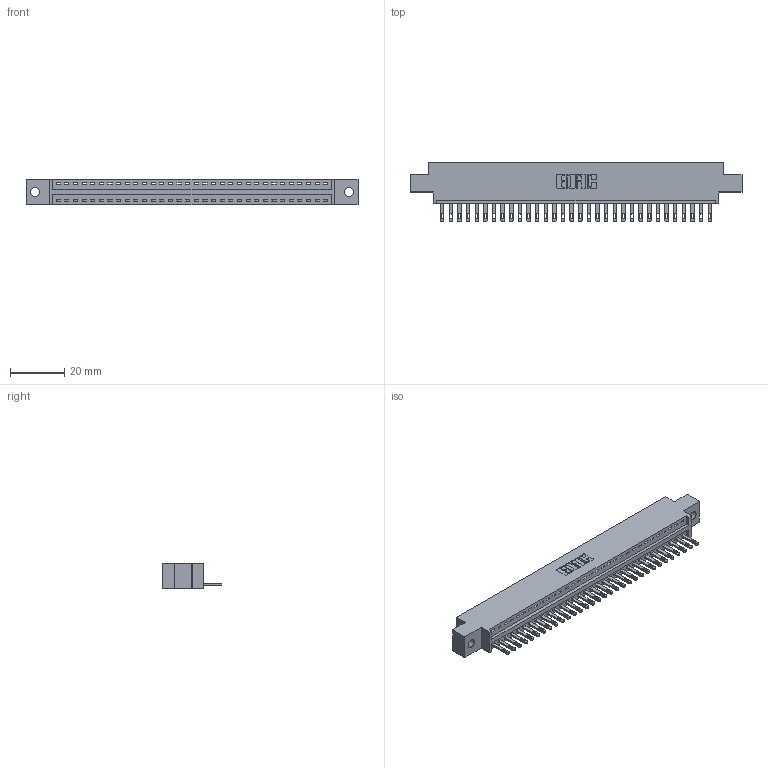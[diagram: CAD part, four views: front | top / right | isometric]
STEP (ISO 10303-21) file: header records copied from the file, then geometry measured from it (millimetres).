
FILE_DESCRIPTION (( 'STEP AP203' ), '1' );
FILE_NAME ('896-032-500-602.STEP', '2021-07-27T19:18:08', ( '' ), ( '' ), 'SwSTEP 2.0', 'SolidWorks 2020', '' );
FILE_SCHEMA (( 'CONFIG_CONTROL_DESIGN' ));
Length unit declared in the file: inch
Products named in the file (3): 846 Part_0.170 Offset - 0.128 Dia; 345-292-001_345-293-100; 896-032-500-602
Assembly tree (33 placements, depth 2):
  896-032-500-602
    846 Part_0.170 Offset - 0.128 Dia
    345-292-001_345-293-100  x32
Bounding box: 122.17 x 21.84 x 9.4 mm (x, y, z)
Volume: 11454.4 mm3; surface area: 14172.2 mm2
Topology: 33 solids, 33 shells, 1854 faces, 5717 edges, 3810 vertices
Faces by surface type: plane 1168, cylinder 686
Entity records: 21271 total; most frequent: CARTESIAN_POINT 3656, ORIENTED_EDGE 3622, DIRECTION 3239, EDGE_CURVE 1811, LINE 1547, VECTOR 1547, VERTEX_POINT 1206, AXIS2_PLACEMENT_3D 846
